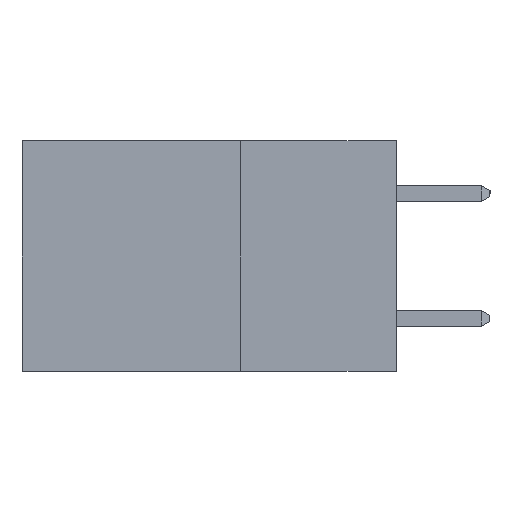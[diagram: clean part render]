
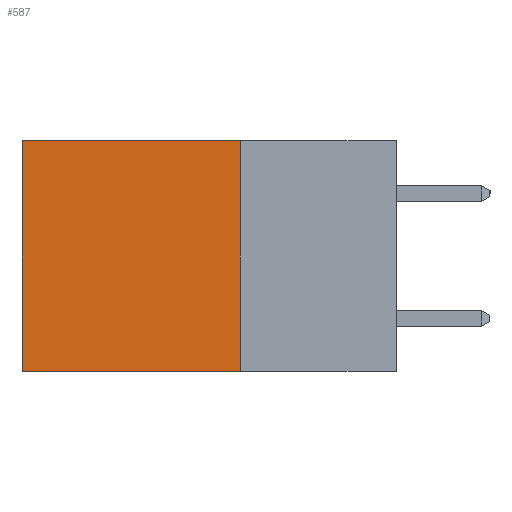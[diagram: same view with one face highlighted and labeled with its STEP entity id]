
A CAD part, left-side view. The second image highlights one B-rep face of the part: STEP entity #587.
In plain terms, the highlighted planar face has unit normal (-1, 0, 0).
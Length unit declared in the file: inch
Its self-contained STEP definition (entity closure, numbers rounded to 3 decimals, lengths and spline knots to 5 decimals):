
#100 = LINE ( 'NONE', #5324, #1203 ) ;
#168 = EDGE_CURVE ( 'NONE', #3222, #8837, #5272, .T. ) ;
#587 = ADVANCED_FACE ( 'NONE', ( #4209 ), #5784, .F. ) ;
#956 = EDGE_CURVE ( 'NONE', #1749, #3222, #5054, .T. ) ;
#1040 = LINE ( 'NONE', #1955, #7412 ) ;
#1203 = VECTOR ( 'NONE', #6234, 39.37008 ) ;
#1642 = ORIENTED_EDGE ( 'NONE', *, *, #6483, .T. ) ;
#1749 = VERTEX_POINT ( 'NONE', #8124 ) ;
#1887 = DIRECTION ( 'NONE',  ( 1., 0., 0. ) ) ;
#1955 = CARTESIAN_POINT ( 'NONE',  ( 0.2615, 0.6, -0.37 ) ) ;
#2004 = DIRECTION ( 'NONE',  ( 0., 0., -1. ) ) ;
#3077 = EDGE_LOOP ( 'NONE', ( #9458, #9421, #8865, #1642 ) ) ;
#3222 = VERTEX_POINT ( 'NONE', #10062 ) ;
#3794 = CARTESIAN_POINT ( 'NONE',  ( 0.2615, 0.25, -0.37 ) ) ;
#3865 = CARTESIAN_POINT ( 'NONE',  ( 0.2615, 0.6, 0. ) ) ;
#4008 = CARTESIAN_POINT ( 'NONE',  ( 0.2615, 0.6, -0.37 ) ) ;
#4209 = FACE_OUTER_BOUND ( 'NONE', #3077, .T. ) ;
#4794 = VECTOR ( 'NONE', #5107, 39.37008 ) ;
#5017 = DIRECTION ( 'NONE',  ( 0., 0., -1. ) ) ;
#5054 = LINE ( 'NONE', #8268, #4794 ) ;
#5107 = DIRECTION ( 'NONE',  ( 0., 0., -1. ) ) ;
#5272 = LINE ( 'NONE', #3794, #9882 ) ;
#5284 = AXIS2_PLACEMENT_3D ( 'NONE', #8892, #1887, #5017 ) ;
#5324 = CARTESIAN_POINT ( 'NONE',  ( 0.2615, 0.25, 0. ) ) ;
#5784 = PLANE ( 'NONE',  #5284 ) ;
#6060 = VERTEX_POINT ( 'NONE', #3865 ) ;
#6234 = DIRECTION ( 'NONE',  ( 0., 1., 0. ) ) ;
#6483 = EDGE_CURVE ( 'NONE', #1749, #6060, #100, .T. ) ;
#7366 = EDGE_CURVE ( 'NONE', #6060, #8837, #1040, .T. ) ;
#7412 = VECTOR ( 'NONE', #2004, 39.37008 ) ;
#8124 = CARTESIAN_POINT ( 'NONE',  ( 0.2615, 0.25, 0. ) ) ;
#8268 = CARTESIAN_POINT ( 'NONE',  ( 0.2615, 0.25, -0.37 ) ) ;
#8529 = DIRECTION ( 'NONE',  ( 0., 1., 0. ) ) ;
#8837 = VERTEX_POINT ( 'NONE', #4008 ) ;
#8865 = ORIENTED_EDGE ( 'NONE', *, *, #956, .F. ) ;
#8892 = CARTESIAN_POINT ( 'NONE',  ( 0.2615, 0.25, -0.37 ) ) ;
#9421 = ORIENTED_EDGE ( 'NONE', *, *, #168, .F. ) ;
#9458 = ORIENTED_EDGE ( 'NONE', *, *, #7366, .T. ) ;
#9882 = VECTOR ( 'NONE', #8529, 39.37008 ) ;
#10062 = CARTESIAN_POINT ( 'NONE',  ( 0.2615, 0.25, -0.37 ) ) ;
